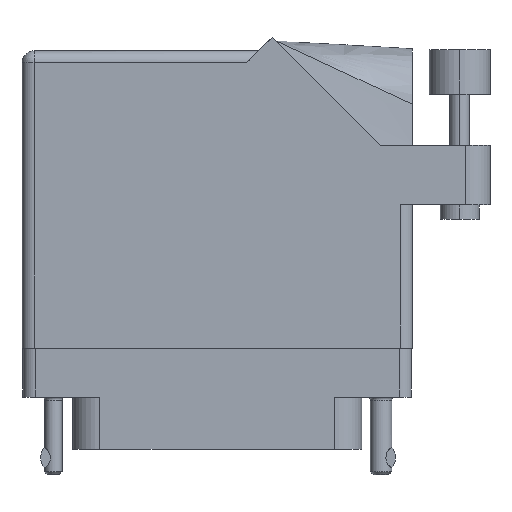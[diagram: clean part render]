
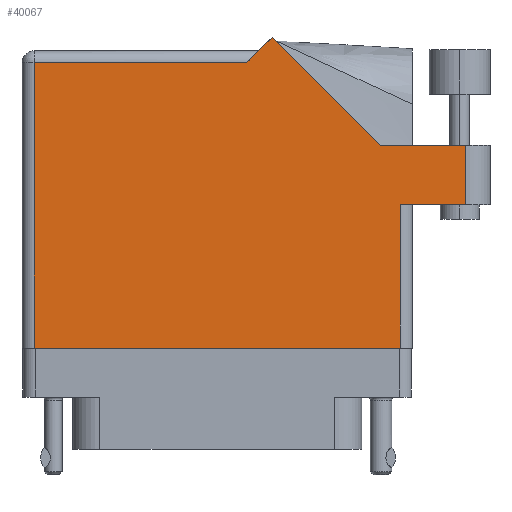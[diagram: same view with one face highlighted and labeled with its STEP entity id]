
A CAD part, front view. The second image highlights one B-rep face of the part: STEP entity #40067.
In plain terms, the highlighted face is planar.
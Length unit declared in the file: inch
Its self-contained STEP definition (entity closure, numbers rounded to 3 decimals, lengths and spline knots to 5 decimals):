
#478 = LINE ( 'NONE', #17796, #48659 ) ;
#577 = CARTESIAN_POINT ( 'NONE',  ( 0.28271, 1.50071, 0.455 ) ) ;
#1567 = AXIS2_PLACEMENT_3D ( 'NONE', #46915, #31259, #12503 ) ;
#2026 = DIRECTION ( 'NONE',  ( 1., 0., 0. ) ) ;
#2594 = DIRECTION ( 'NONE',  ( -1., 0., 0. ) ) ;
#4656 = CARTESIAN_POINT ( 'NONE',  ( 1.28, 0.944, 0.455 ) ) ;
#5302 = CARTESIAN_POINT ( 'NONE',  ( 1.005, 0.637, 0.455 ) ) ;
#5399 = EDGE_LOOP ( 'NONE', ( #44525, #27490, #44136, #33988, #37406, #8572, #24763, #35141, #13214 ) ) ;
#5634 = CARTESIAN_POINT ( 'NONE',  ( 1.28, 0.944, 0.455 ) ) ;
#6299 = EDGE_CURVE ( 'NONE', #30467, #12160, #47055, .T. ) ;
#6723 = CARTESIAN_POINT ( 'NONE',  ( -0.943, -0.1, 0.455 ) ) ;
#7301 = LINE ( 'NONE', #27907, #40564 ) ;
#8149 = VERTEX_POINT ( 'NONE', #13223 ) ;
#8315 = CARTESIAN_POINT ( 'NONE',  ( 0.943, 0.637, 0.455 ) ) ;
#8572 = ORIENTED_EDGE ( 'NONE', *, *, #33330, .T. ) ;
#9161 = FACE_OUTER_BOUND ( 'NONE', #5399, .T. ) ;
#10079 = VERTEX_POINT ( 'NONE', #12441 ) ;
#11454 = DIRECTION ( 'NONE',  ( -0.707, 0.707, 0. ) ) ;
#11745 = EDGE_CURVE ( 'NONE', #27197, #24959, #30743, .T. ) ;
#12154 = LINE ( 'NONE', #5302, #40683 ) ;
#12160 = VERTEX_POINT ( 'NONE', #8315 ) ;
#12441 = CARTESIAN_POINT ( 'NONE',  ( -0.943, 1.368, 0.455 ) ) ;
#12503 = DIRECTION ( 'NONE',  ( -1., 0., 0. ) ) ;
#12806 = CARTESIAN_POINT ( 'NONE',  ( 0.943, -0.1, 0.455 ) ) ;
#12943 = DIRECTION ( 'NONE',  ( 1., 0., 0. ) ) ;
#13214 = ORIENTED_EDGE ( 'NONE', *, *, #6299, .T. ) ;
#13223 = CARTESIAN_POINT ( 'NONE',  ( 0.15, 1.368, 0.455 ) ) ;
#13706 = CARTESIAN_POINT ( 'NONE',  ( 0.943, 0.637, 0.455 ) ) ;
#17297 = VECTOR ( 'NONE', #11454, 39.37008 ) ;
#17796 = CARTESIAN_POINT ( 'NONE',  ( -1.005, 1.368, 0.455 ) ) ;
#18324 = DIRECTION ( 'NONE',  ( 0., 1., 0. ) ) ;
#20394 = LINE ( 'NONE', #37451, #29311 ) ;
#20546 = EDGE_CURVE ( 'NONE', #42711, #8149, #20394, .T. ) ;
#20647 = DIRECTION ( 'NONE',  ( 0., -1., 0. ) ) ;
#21809 = VERTEX_POINT ( 'NONE', #44638 ) ;
#22228 = EDGE_CURVE ( 'NONE', #24959, #21809, #7301, .T. ) ;
#23259 = VERTEX_POINT ( 'NONE', #6723 ) ;
#24298 = LINE ( 'NONE', #36742, #26670 ) ;
#24763 = ORIENTED_EDGE ( 'NONE', *, *, #41004, .T. ) ;
#24959 = VERTEX_POINT ( 'NONE', #5634 ) ;
#26670 = VECTOR ( 'NONE', #2026, 39.37008 ) ;
#27197 = VERTEX_POINT ( 'NONE', #36528 ) ;
#27490 = ORIENTED_EDGE ( 'NONE', *, *, #11745, .T. ) ;
#27535 = DIRECTION ( 'NONE',  ( 0., 1., 0. ) ) ;
#27907 = CARTESIAN_POINT ( 'NONE',  ( 1.405, 0.944, 0.455 ) ) ;
#29311 = VECTOR ( 'NONE', #41256, 39.37008 ) ;
#30467 = VERTEX_POINT ( 'NONE', #12806 ) ;
#30743 = LINE ( 'NONE', #4656, #34312 ) ;
#31259 = DIRECTION ( 'NONE',  ( 0., 0., -1. ) ) ;
#32100 = DIRECTION ( 'NONE',  ( -1., 0., 0. ) ) ;
#32251 = LINE ( 'NONE', #43455, #45366 ) ;
#33330 = EDGE_CURVE ( 'NONE', #8149, #10079, #478, .T. ) ;
#33369 = LINE ( 'NONE', #34181, #17297 ) ;
#33796 = EDGE_CURVE ( 'NONE', #21809, #42711, #33369, .T. ) ;
#33988 = ORIENTED_EDGE ( 'NONE', *, *, #33796, .T. ) ;
#34181 = CARTESIAN_POINT ( 'NONE',  ( 0.83942, 0.944, 0.455 ) ) ;
#34312 = VECTOR ( 'NONE', #27535, 39.37008 ) ;
#35058 = EDGE_CURVE ( 'NONE', #23259, #30467, #24298, .T. ) ;
#35141 = ORIENTED_EDGE ( 'NONE', *, *, #35058, .T. ) ;
#35730 = VECTOR ( 'NONE', #18324, 39.37008 ) ;
#36528 = CARTESIAN_POINT ( 'NONE',  ( 1.28, 0.637, 0.455 ) ) ;
#36742 = CARTESIAN_POINT ( 'NONE',  ( -1.005, -0.1, 0.455 ) ) ;
#37406 = ORIENTED_EDGE ( 'NONE', *, *, #20546, .T. ) ;
#37451 = CARTESIAN_POINT ( 'NONE',  ( 0.212, 1.43, 0.455 ) ) ;
#39278 = PLANE ( 'NONE',  #1567 ) ;
#40067 = ADVANCED_FACE ( 'NONE', ( #9161 ), #39278, .F. ) ;
#40564 = VECTOR ( 'NONE', #32100, 39.37008 ) ;
#40683 = VECTOR ( 'NONE', #12943, 39.37008 ) ;
#41004 = EDGE_CURVE ( 'NONE', #10079, #23259, #32251, .T. ) ;
#41256 = DIRECTION ( 'NONE',  ( -0.707, -0.707, 0. ) ) ;
#41967 = EDGE_CURVE ( 'NONE', #12160, #27197, #12154, .T. ) ;
#42711 = VERTEX_POINT ( 'NONE', #577 ) ;
#43455 = CARTESIAN_POINT ( 'NONE',  ( -0.943, -0.1, 0.455 ) ) ;
#44136 = ORIENTED_EDGE ( 'NONE', *, *, #22228, .T. ) ;
#44525 = ORIENTED_EDGE ( 'NONE', *, *, #41967, .T. ) ;
#44638 = CARTESIAN_POINT ( 'NONE',  ( 0.83942, 0.944, 0.455 ) ) ;
#45366 = VECTOR ( 'NONE', #20647, 39.37008 ) ;
#46915 = CARTESIAN_POINT ( 'NONE',  ( -1.005, 1.43, 0.455 ) ) ;
#47055 = LINE ( 'NONE', #13706, #35730 ) ;
#48659 = VECTOR ( 'NONE', #2594, 39.37008 ) ;
